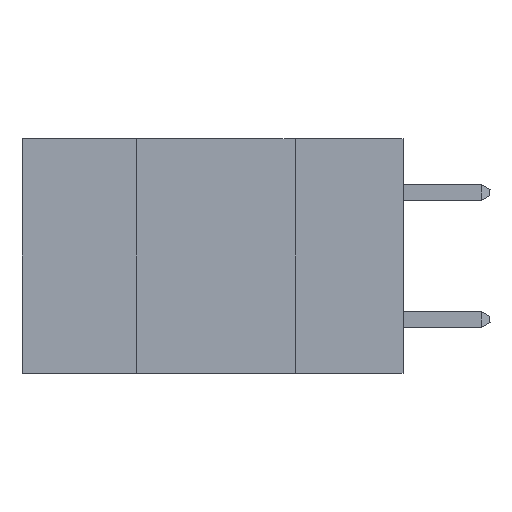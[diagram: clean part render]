
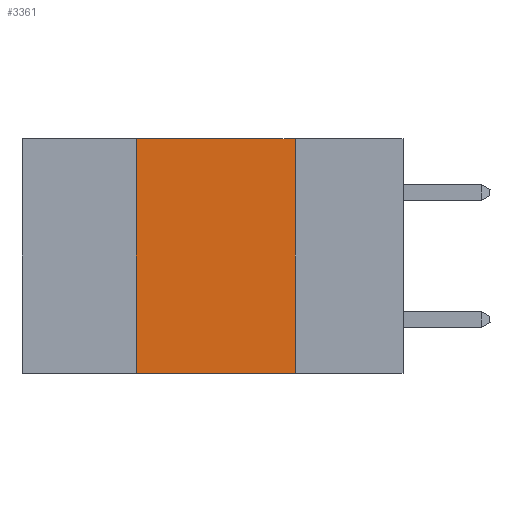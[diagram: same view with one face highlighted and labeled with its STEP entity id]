
A CAD part, left-side view. The second image highlights one B-rep face of the part: STEP entity #3361.
In plain terms, the highlighted planar face has unit normal (-1, 0, 0).
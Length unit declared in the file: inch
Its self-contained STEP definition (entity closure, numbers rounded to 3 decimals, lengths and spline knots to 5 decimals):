
#1256 = ORIENTED_EDGE ( 'NONE', *, *, #2526, .T. ) ;
#1747 = EDGE_CURVE ( 'NONE', #2473, #17384, #4410, .T. ) ;
#1902 = CARTESIAN_POINT ( 'NONE',  ( 0., 0.6, 0. ) ) ;
#2473 = VERTEX_POINT ( 'NONE', #9533 ) ;
#2526 = EDGE_CURVE ( 'NONE', #9544, #17384, #7868, .T. ) ;
#3065 = DIRECTION ( 'NONE',  ( 0., 0., -1. ) ) ;
#3361 = ADVANCED_FACE ( 'NONE', ( #16739 ), #14919, .F. ) ;
#3917 = VECTOR ( 'NONE', #4259, 39.37008 ) ;
#4259 = DIRECTION ( 'NONE',  ( 0., -1., 0. ) ) ;
#4410 = LINE ( 'NONE', #17813, #7441 ) ;
#4450 = ORIENTED_EDGE ( 'NONE', *, *, #6168, .F. ) ;
#4658 = CARTESIAN_POINT ( 'NONE',  ( 0., 0.6, -0.37 ) ) ;
#5507 = VECTOR ( 'NONE', #10853, 39.37008 ) ;
#5906 = AXIS2_PLACEMENT_3D ( 'NONE', #7507, #12018, #3065 ) ;
#6168 = EDGE_CURVE ( 'NONE', #9544, #19158, #14573, .T. ) ;
#6603 = VECTOR ( 'NONE', #11288, 39.37008 ) ;
#7244 = EDGE_LOOP ( 'NONE', ( #11776, #14526, #4450, #1256 ) ) ;
#7441 = VECTOR ( 'NONE', #8127, 39.37008 ) ;
#7507 = CARTESIAN_POINT ( 'NONE',  ( 0., 0.6, 0. ) ) ;
#7868 = LINE ( 'NONE', #4658, #3917 ) ;
#8127 = DIRECTION ( 'NONE',  ( 0., 0., -1. ) ) ;
#9533 = CARTESIAN_POINT ( 'NONE',  ( 0., 0.17, 0. ) ) ;
#9544 = VERTEX_POINT ( 'NONE', #16013 ) ;
#9758 = CARTESIAN_POINT ( 'NONE',  ( 0., 0.42, 0. ) ) ;
#10853 = DIRECTION ( 'NONE',  ( 0., -1., 0. ) ) ;
#11288 = DIRECTION ( 'NONE',  ( 0., 0., 1. ) ) ;
#11776 = ORIENTED_EDGE ( 'NONE', *, *, #1747, .F. ) ;
#11852 = EDGE_CURVE ( 'NONE', #19158, #2473, #13431, .T. ) ;
#12018 = DIRECTION ( 'NONE',  ( 1., 0., 0. ) ) ;
#13431 = LINE ( 'NONE', #1902, #5507 ) ;
#14526 = ORIENTED_EDGE ( 'NONE', *, *, #11852, .F. ) ;
#14573 = LINE ( 'NONE', #9758, #6603 ) ;
#14919 = PLANE ( 'NONE',  #5906 ) ;
#14953 = CARTESIAN_POINT ( 'NONE',  ( 0., 0.17, -0.37 ) ) ;
#16013 = CARTESIAN_POINT ( 'NONE',  ( 0., 0.42, -0.37 ) ) ;
#16349 = CARTESIAN_POINT ( 'NONE',  ( 0., 0.42, 0. ) ) ;
#16739 = FACE_OUTER_BOUND ( 'NONE', #7244, .T. ) ;
#17384 = VERTEX_POINT ( 'NONE', #14953 ) ;
#17813 = CARTESIAN_POINT ( 'NONE',  ( 0., 0.17, 0. ) ) ;
#19158 = VERTEX_POINT ( 'NONE', #16349 ) ;
